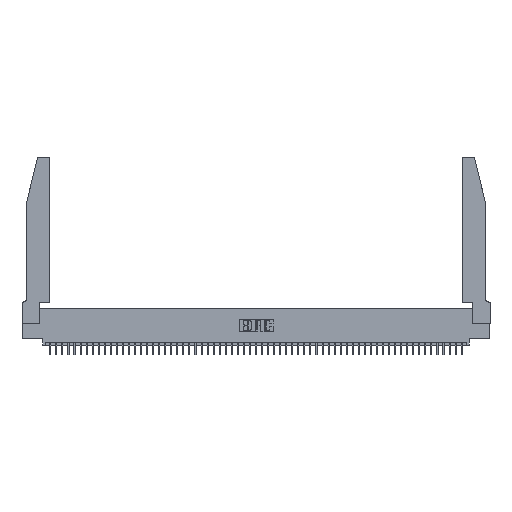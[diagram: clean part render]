
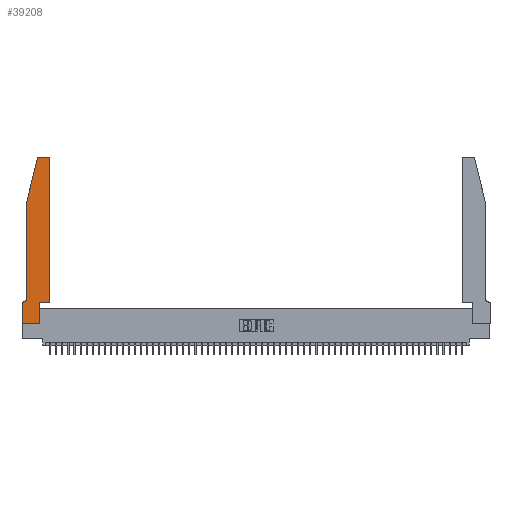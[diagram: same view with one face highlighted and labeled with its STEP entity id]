
A CAD part, top view. The second image highlights one B-rep face of the part: STEP entity #39208.
In plain terms, the highlighted planar face has unit normal (0, 0, 1).
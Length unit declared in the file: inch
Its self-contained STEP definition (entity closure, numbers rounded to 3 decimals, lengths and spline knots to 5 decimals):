
#19 = ORIENTED_EDGE ( 'NONE', *, *, #36211, .T. ) ;
#37 = CARTESIAN_POINT ( 'NONE',  ( 0.0755, 2., 0.37 ) ) ;
#653 = AXIS2_PLACEMENT_3D ( 'NONE', #48337, #22675, #52575 ) ;
#1891 = VERTEX_POINT ( 'NONE', #18761 ) ;
#2989 = AXIS2_PLACEMENT_3D ( 'NONE', #50838, #25248, #55098 ) ;
#3887 = CARTESIAN_POINT ( 'NONE',  ( 0.4505, 2.72, 0.37 ) ) ;
#4062 = VECTOR ( 'NONE', #4416, 39.37008 ) ;
#4416 = DIRECTION ( 'NONE',  ( -0.239, -0.971, 0. ) ) ;
#4775 = LINE ( 'NONE', #30878, #24940 ) ;
#6451 = DIRECTION ( 'NONE',  ( 0., 1., 0. ) ) ;
#6583 = VECTOR ( 'NONE', #54308, 39.37008 ) ;
#6653 = ORIENTED_EDGE ( 'NONE', *, *, #46246, .T. ) ;
#7439 = VERTEX_POINT ( 'NONE', #33220 ) ;
#10664 = CARTESIAN_POINT ( 'NONE',  ( 0.0055, 0.42, 0.37 ) ) ;
#10778 = CIRCLE ( 'NONE', #15519, 0.07 ) ;
#11262 = CARTESIAN_POINT ( 'NONE',  ( 0.284, 2.75, 0.37 ) ) ;
#12373 = VECTOR ( 'NONE', #50947, 39.37008 ) ;
#12683 = EDGE_CURVE ( 'NONE', #36258, #13315, #53155, .T. ) ;
#13315 = VERTEX_POINT ( 'NONE', #19835 ) ;
#13325 = CARTESIAN_POINT ( 'NONE',  ( 0., 0., 0.37 ) ) ;
#14880 = EDGE_CURVE ( 'NONE', #1891, #44455, #4775, .T. ) ;
#14989 = DIRECTION ( 'NONE',  ( -1., 0., 0. ) ) ;
#15071 = EDGE_CURVE ( 'NONE', #44801, #50383, #26953, .T. ) ;
#15505 = ORIENTED_EDGE ( 'NONE', *, *, #14880, .T. ) ;
#15519 = AXIS2_PLACEMENT_3D ( 'NONE', #10664, #40679, #14989 ) ;
#16253 = CIRCLE ( 'NONE', #45680, 0.03 ) ;
#17639 = DIRECTION ( 'NONE',  ( 1., 0., 0. ) ) ;
#18761 = CARTESIAN_POINT ( 'NONE',  ( 0., 0.35, 0.37 ) ) ;
#18768 = VERTEX_POINT ( 'NONE', #11262 ) ;
#18851 = CARTESIAN_POINT ( 'NONE',  ( 0.0755, 2., 0.37 ) ) ;
#18903 = CARTESIAN_POINT ( 'NONE',  ( 0.2605, 2.75, 0.37 ) ) ;
#19348 = LINE ( 'NONE', #32263, #53471 ) ;
#19835 = CARTESIAN_POINT ( 'NONE',  ( 0.4505, 0.35, 0.37 ) ) ;
#20985 = DIRECTION ( 'NONE',  ( 0., 0., 1. ) ) ;
#22403 = ORIENTED_EDGE ( 'NONE', *, *, #25204, .T. ) ;
#22620 = EDGE_LOOP ( 'NONE', ( #25728, #55298, #55272, #19, #27121, #49225, #15505, #22403, #6653, #24157, #36284, #25771 ) ) ;
#22675 = DIRECTION ( 'NONE',  ( 0., 0., 1. ) ) ;
#23791 = LINE ( 'NONE', #42390, #12373 ) ;
#24157 = ORIENTED_EDGE ( 'NONE', *, *, #12683, .T. ) ;
#24559 = CARTESIAN_POINT ( 'NONE',  ( 0.0055, 0.35, 0.37 ) ) ;
#24818 = CARTESIAN_POINT ( 'NONE',  ( 0.4205, 2.75, 0.37 ) ) ;
#24940 = VECTOR ( 'NONE', #35169, 39.37008 ) ;
#25204 = EDGE_CURVE ( 'NONE', #44455, #7439, #35425, .T. ) ;
#25248 = DIRECTION ( 'NONE',  ( 0., 0., 1. ) ) ;
#25722 = VECTOR ( 'NONE', #53130, 39.37008 ) ;
#25728 = ORIENTED_EDGE ( 'NONE', *, *, #35163, .T. ) ;
#25771 = ORIENTED_EDGE ( 'NONE', *, *, #35058, .T. ) ;
#26953 = LINE ( 'NONE', #37, #4062 ) ;
#27121 = ORIENTED_EDGE ( 'NONE', *, *, #36361, .T. ) ;
#29939 = DIRECTION ( 'NONE',  ( 0., -1., 0. ) ) ;
#30878 = CARTESIAN_POINT ( 'NONE',  ( 0., 0., 0.37 ) ) ;
#32263 = CARTESIAN_POINT ( 'NONE',  ( 0.4505, 0.35, 0.37 ) ) ;
#32644 = CARTESIAN_POINT ( 'NONE',  ( 0.0755, 0.42, 0.37 ) ) ;
#33047 = CARTESIAN_POINT ( 'NONE',  ( 0.25487, 2.72718, 0.37 ) ) ;
#33220 = CARTESIAN_POINT ( 'NONE',  ( 0.2865, 0., 0.37 ) ) ;
#34473 = CARTESIAN_POINT ( 'NONE',  ( 0.2865, 0.35, 0.37 ) ) ;
#35058 = EDGE_CURVE ( 'NONE', #38565, #51157, #52431, .T. ) ;
#35163 = EDGE_CURVE ( 'NONE', #51157, #18768, #39811, .T. ) ;
#35169 = DIRECTION ( 'NONE',  ( 0., -1., 0. ) ) ;
#35425 = LINE ( 'NONE', #39034, #55346 ) ;
#36211 = EDGE_CURVE ( 'NONE', #50383, #54001, #50322, .T. ) ;
#36258 = VERTEX_POINT ( 'NONE', #34473 ) ;
#36284 = ORIENTED_EDGE ( 'NONE', *, *, #38936, .T. ) ;
#36361 = EDGE_CURVE ( 'NONE', #54001, #51561, #10778, .T. ) ;
#38565 = VERTEX_POINT ( 'NONE', #3887 ) ;
#38936 = EDGE_CURVE ( 'NONE', #13315, #38565, #19348, .T. ) ;
#39022 = VECTOR ( 'NONE', #29939, 39.37008 ) ;
#39034 = CARTESIAN_POINT ( 'NONE',  ( 0., 0., 0.37 ) ) ;
#39208 = ADVANCED_FACE ( 'NONE', ( #51461 ), #42282, .T. ) ;
#39811 = LINE ( 'NONE', #18903, #25722 ) ;
#40679 = DIRECTION ( 'NONE',  ( 0., 0., -1. ) ) ;
#40842 = LINE ( 'NONE', #50052, #6583 ) ;
#40936 = CARTESIAN_POINT ( 'NONE',  ( 0.4505, 0.35, 0.37 ) ) ;
#42282 = PLANE ( 'NONE',  #2989 ) ;
#42390 = CARTESIAN_POINT ( 'NONE',  ( 0.2865, 0.35, 0.37 ) ) ;
#44455 = VERTEX_POINT ( 'NONE', #13325 ) ;
#44801 = VERTEX_POINT ( 'NONE', #33047 ) ;
#45680 = AXIS2_PLACEMENT_3D ( 'NONE', #46606, #20985, #50890 ) ;
#46246 = EDGE_CURVE ( 'NONE', #7439, #36258, #23791, .T. ) ;
#46606 = CARTESIAN_POINT ( 'NONE',  ( 0.284, 2.72, 0.37 ) ) ;
#46900 = CARTESIAN_POINT ( 'NONE',  ( 0.0755, 2., 0.37 ) ) ;
#48337 = CARTESIAN_POINT ( 'NONE',  ( 0.4205, 2.72, 0.37 ) ) ;
#49225 = ORIENTED_EDGE ( 'NONE', *, *, #52717, .T. ) ;
#50033 = EDGE_CURVE ( 'NONE', #18768, #44801, #16253, .T. ) ;
#50052 = CARTESIAN_POINT ( 'NONE',  ( 0.0755, 0.35, 0.37 ) ) ;
#50322 = LINE ( 'NONE', #46900, #39022 ) ;
#50383 = VERTEX_POINT ( 'NONE', #18851 ) ;
#50838 = CARTESIAN_POINT ( 'NONE',  ( 0., 0.35, 0.37 ) ) ;
#50890 = DIRECTION ( 'NONE',  ( 1., 0., 0. ) ) ;
#50947 = DIRECTION ( 'NONE',  ( 0., 1., 0. ) ) ;
#51157 = VERTEX_POINT ( 'NONE', #24818 ) ;
#51461 = FACE_OUTER_BOUND ( 'NONE', #22620, .T. ) ;
#51561 = VERTEX_POINT ( 'NONE', #24559 ) ;
#51810 = VECTOR ( 'NONE', #53762, 39.37008 ) ;
#52431 = CIRCLE ( 'NONE', #653, 0.03 ) ;
#52575 = DIRECTION ( 'NONE',  ( 1., 0., 0. ) ) ;
#52717 = EDGE_CURVE ( 'NONE', #51561, #1891, #40842, .T. ) ;
#53130 = DIRECTION ( 'NONE',  ( -1., 0., 0. ) ) ;
#53155 = LINE ( 'NONE', #40936, #51810 ) ;
#53471 = VECTOR ( 'NONE', #6451, 39.37008 ) ;
#53762 = DIRECTION ( 'NONE',  ( 1., 0., 0. ) ) ;
#54001 = VERTEX_POINT ( 'NONE', #32644 ) ;
#54308 = DIRECTION ( 'NONE',  ( -1., 0., 0. ) ) ;
#55098 = DIRECTION ( 'NONE',  ( 1., 0., 0. ) ) ;
#55272 = ORIENTED_EDGE ( 'NONE', *, *, #15071, .T. ) ;
#55298 = ORIENTED_EDGE ( 'NONE', *, *, #50033, .T. ) ;
#55346 = VECTOR ( 'NONE', #17639, 39.37008 ) ;
